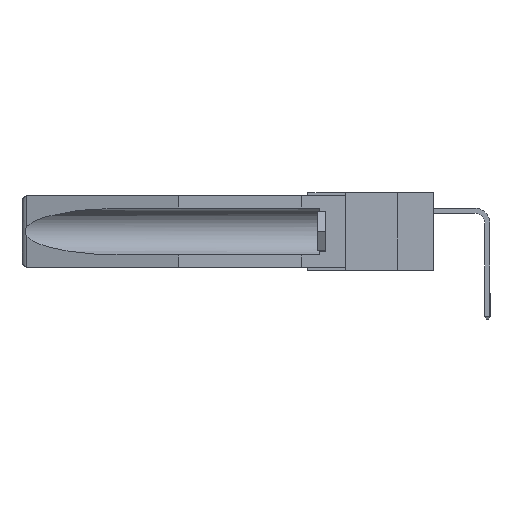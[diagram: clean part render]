
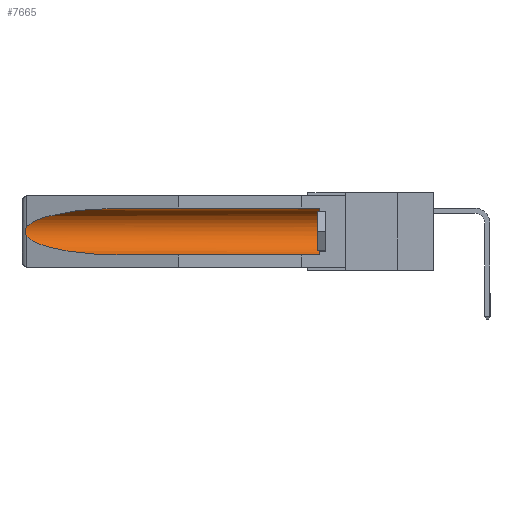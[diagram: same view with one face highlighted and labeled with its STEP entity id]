
A CAD part, left-side view. The second image highlights one B-rep face of the part: STEP entity #7665.
In plain terms, the highlighted cylindrical face has radius 2.857 mm (diameter 5.715 mm), a partial arc.
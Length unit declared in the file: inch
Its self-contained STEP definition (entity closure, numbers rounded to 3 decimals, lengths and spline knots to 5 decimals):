
#504 = CARTESIAN_POINT ( 'NONE',  ( 0.155, -0.30754, -0.284 ) ) ;
#2365 = DIRECTION ( 'NONE',  ( 0., 0., 1. ) ) ;
#3212 = EDGE_LOOP ( 'NONE', ( #5442, #21360, #15421, #16712, #23003, #16602 ) ) ;
#3670 = EDGE_CURVE ( 'NONE', #9057, #14892, #23418, .T. ) ;
#3717 = CARTESIAN_POINT ( 'NONE',  ( 0.21114, 1.30732, -0.284 ) ) ;
#3838 = CARTESIAN_POINT ( 'NONE',  ( 0.2675, 1.53308, -0.17534 ) ) ;
#4759 = CARTESIAN_POINT ( 'NONE',  ( 0.155, 0.126, -0.284 ) ) ;
#5381 = CARTESIAN_POINT ( 'NONE',  ( 0.26537, 1.52718, -0.14972 ) ) ;
#5442 = ORIENTED_EDGE ( 'NONE', *, *, #15238, .T. ) ;
#6409 = VERTEX_POINT ( 'NONE', #4759 ) ;
#6492 = DIRECTION ( 'NONE',  ( 0., 1., 0. ) ) ;
#6548 = VECTOR ( 'NONE', #23321, 39.37008 ) ;
#6573 = DIRECTION ( 'NONE',  ( 0., 0., 1. ) ) ;
#6627 = CARTESIAN_POINT ( 'NONE',  ( 0.26537, 1.52718, -0.19328 ) ) ;
#6836 = CARTESIAN_POINT ( 'NONE',  ( 0.155, 1.07973, -0.059 ) ) ;
#6924 = VERTEX_POINT ( 'NONE', #12216 ) ;
#7019 = VERTEX_POINT ( 'NONE', #21697 ) ;
#7197 = CARTESIAN_POINT ( 'NONE',  ( 0.2673, 1.5327, -0.16383 ) ) ;
#7478 = CARTESIAN_POINT ( 'NONE',  ( 0.25451, 1.48313, -0.24835 ) ) ;
#7665 = ADVANCED_FACE ( 'NONE', ( #18842 ), #17673, .F. ) ;
#9057 = VERTEX_POINT ( 'NONE', #6627 ) ;
#9139 = EDGE_CURVE ( 'NONE', #7019, #18206, #11512, .T. ) ;
#9204 = LINE ( 'NONE', #504, #21106 ) ;
#9713 = CARTESIAN_POINT ( 'NONE',  ( 0.25451, 1.48313, -0.09465 ) ) ;
#10460 = CARTESIAN_POINT ( 'NONE',  ( 0.155, -0.30754, -0.059 ) ) ;
#10628 = AXIS2_PLACEMENT_3D ( 'NONE', #15304, #21127, #2365 ) ;
#11019 = CARTESIAN_POINT ( 'NONE',  ( 0.2675, 1.53308, -0.16763 ) ) ;
#11093 = CARTESIAN_POINT ( 'NONE',  ( 0.2673, 1.53269, -0.17917 ) ) ;
#11295 = CARTESIAN_POINT ( 'NONE',  ( 0.26537, 1.52718, -0.19328 ) ) ;
#11375 = CARTESIAN_POINT ( 'NONE',  ( 0.155, 1.07973, -0.284 ) ) ;
#11512 = LINE ( 'NONE', #10460, #6548 ) ;
#11816 = B_SPLINE_CURVE_WITH_KNOTS ( 'NONE', 3,
 ( #5381, #22190, #22113, #7197, #11019, #3838, #11093, #24043, #22041, #23963 ),
 .UNSPECIFIED., .F., .F.,
 ( 4, 2, 2, 2, 4 ),
 ( 0., 0.00029, 0.00058, 0.00087, 0.00117 ),
 .UNSPECIFIED. ) ;
#12216 = CARTESIAN_POINT ( 'NONE',  ( 0.26537, 1.52718, -0.14972 ) ) ;
#12844 = CARTESIAN_POINT ( 'NONE',  ( 0.155, 1.07973, -0.284 ) ) ;
#13198 = AXIS2_PLACEMENT_3D ( 'NONE', #17609, #6492, #6573 ) ;
#13529 = DIRECTION ( 'NONE',  ( 0., 1., 0. ) ) ;
#13850 = CARTESIAN_POINT ( 'NONE',  ( 0.26537, 1.52718, -0.14972 ) ) ;
#14680 =( BOUNDED_CURVE ( )  B_SPLINE_CURVE ( 3, ( #20747, #15092, #9713, #13850 ),
 .UNSPECIFIED., .F., .F. ) 
 B_SPLINE_CURVE_WITH_KNOTS ( ( 4, 4 ),
 ( 4.71239, 6.08839 ),
 .UNSPECIFIED. ) 
 CURVE ( )  GEOMETRIC_REPRESENTATION_ITEM ( )  RATIONAL_B_SPLINE_CURVE ( ( 1., 0.848, 0.848, 1. ) ) 
 REPRESENTATION_ITEM ( '' )  );
#14892 = VERTEX_POINT ( 'NONE', #11375 ) ;
#15092 = CARTESIAN_POINT ( 'NONE',  ( 0.21114, 1.30732, -0.059 ) ) ;
#15238 = EDGE_CURVE ( 'NONE', #18206, #6924, #14680, .T. ) ;
#15304 = CARTESIAN_POINT ( 'NONE',  ( 0.155, 0.126, -0.1715 ) ) ;
#15421 = ORIENTED_EDGE ( 'NONE', *, *, #3670, .T. ) ;
#16602 = ORIENTED_EDGE ( 'NONE', *, *, #9139, .T. ) ;
#16712 = ORIENTED_EDGE ( 'NONE', *, *, #20880, .F. ) ;
#16738 = CIRCLE ( 'NONE', #10628, 0.1125 ) ;
#17609 = CARTESIAN_POINT ( 'NONE',  ( 0.155, -0.30754, -0.1715 ) ) ;
#17673 = CYLINDRICAL_SURFACE ( 'NONE', #13198, 0.1125 ) ;
#18206 = VERTEX_POINT ( 'NONE', #6836 ) ;
#18842 = FACE_OUTER_BOUND ( 'NONE', #3212, .T. ) ;
#19395 = EDGE_CURVE ( 'NONE', #6924, #9057, #11816, .T. ) ;
#20747 = CARTESIAN_POINT ( 'NONE',  ( 0.155, 1.07973, -0.059 ) ) ;
#20880 = EDGE_CURVE ( 'NONE', #6409, #14892, #9204, .T. ) ;
#21106 = VECTOR ( 'NONE', #13529, 39.37008 ) ;
#21127 = DIRECTION ( 'NONE',  ( 0., -1., 0. ) ) ;
#21360 = ORIENTED_EDGE ( 'NONE', *, *, #19395, .T. ) ;
#21442 = EDGE_CURVE ( 'NONE', #6409, #7019, #16738, .T. ) ;
#21697 = CARTESIAN_POINT ( 'NONE',  ( 0.155, 0.126, -0.059 ) ) ;
#22041 = CARTESIAN_POINT ( 'NONE',  ( 0.26597, 1.5296, -0.19026 ) ) ;
#22113 = CARTESIAN_POINT ( 'NONE',  ( 0.26654, 1.53092, -0.15636 ) ) ;
#22190 = CARTESIAN_POINT ( 'NONE',  ( 0.26597, 1.52961, -0.15275 ) ) ;
#23003 = ORIENTED_EDGE ( 'NONE', *, *, #21442, .T. ) ;
#23321 = DIRECTION ( 'NONE',  ( 0., 1., 0. ) ) ;
#23418 =( BOUNDED_CURVE ( )  B_SPLINE_CURVE ( 3, ( #11295, #7478, #3717, #12844 ),
 .UNSPECIFIED., .F., .F. ) 
 B_SPLINE_CURVE_WITH_KNOTS ( ( 4, 4 ),
 ( 0.1948, 1.5708 ),
 .UNSPECIFIED. ) 
 CURVE ( )  GEOMETRIC_REPRESENTATION_ITEM ( )  RATIONAL_B_SPLINE_CURVE ( ( 1., 0.848, 0.848, 1. ) ) 
 REPRESENTATION_ITEM ( '' )  );
#23963 = CARTESIAN_POINT ( 'NONE',  ( 0.26537, 1.52718, -0.19328 ) ) ;
#24043 = CARTESIAN_POINT ( 'NONE',  ( 0.26655, 1.53094, -0.18657 ) ) ;
